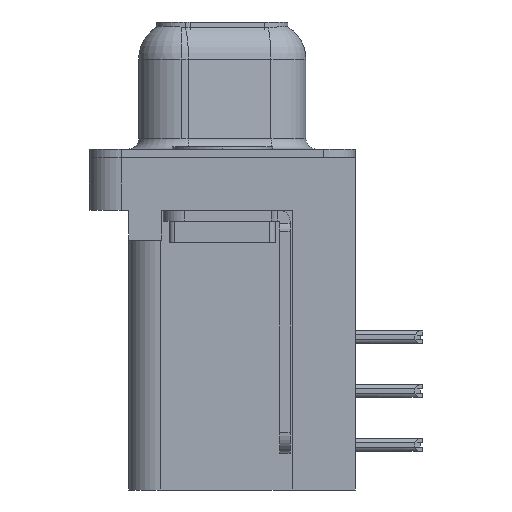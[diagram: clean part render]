
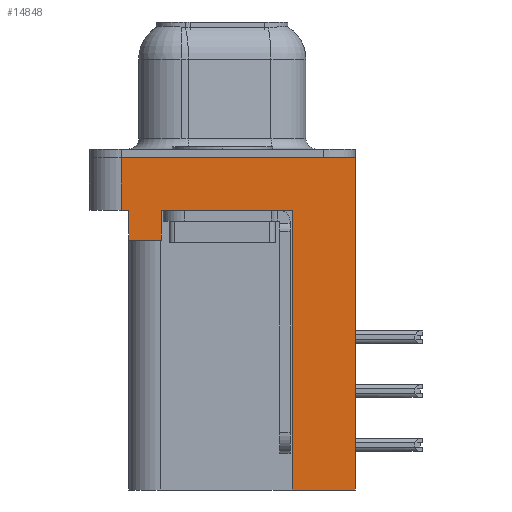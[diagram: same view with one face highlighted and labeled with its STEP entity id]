
A CAD part, left-side view. The second image highlights one B-rep face of the part: STEP entity #14848.
In plain terms, the highlighted planar face has unit normal (-1, 0, 0).
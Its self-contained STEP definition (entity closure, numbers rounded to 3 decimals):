
#446 = VECTOR ( 'NONE', #33375, 1000. ) ;
#2451 = DIRECTION ( 'NONE',  ( 0., 1., 0. ) ) ;
#3460 = ORIENTED_EDGE ( 'NONE', *, *, #33896, .F. ) ;
#3939 = DIRECTION ( 'NONE',  ( 0., 0., 1. ) ) ;
#4551 = CARTESIAN_POINT ( 'NONE',  ( -2.935, 4.425, -3.9 ) ) ;
#4789 = CARTESIAN_POINT ( 'NONE',  ( -2.935, -3.295, -15.7 ) ) ;
#4794 = EDGE_LOOP ( 'NONE', ( #4999, #20649, #5176, #29554, #32400, #23883, #32715, #3460, #33951, #23273 ) ) ;
#4872 = VECTOR ( 'NONE', #16156, 1000. ) ;
#4999 = ORIENTED_EDGE ( 'NONE', *, *, #17273, .F. ) ;
#5027 = AXIS2_PLACEMENT_3D ( 'NONE', #14839, #20171, #3939 ) ;
#5176 = ORIENTED_EDGE ( 'NONE', *, *, #31374, .T. ) ;
#6061 = VECTOR ( 'NONE', #17089, 1000. ) ;
#7099 = VECTOR ( 'NONE', #20869, 1000. ) ;
#8387 = CARTESIAN_POINT ( 'NONE',  ( -2.935, 2.895, -3.9 ) ) ;
#9916 = VECTOR ( 'NONE', #16179, 1000. ) ;
#9974 = DIRECTION ( 'NONE',  ( 0., 0., 1. ) ) ;
#12251 = VECTOR ( 'NONE', #33177, 1000. ) ;
#14275 = CARTESIAN_POINT ( 'NONE',  ( -2.935, 4.775, -2.5 ) ) ;
#14746 = LINE ( 'NONE', #4789, #27880 ) ;
#14839 = CARTESIAN_POINT ( 'NONE',  ( -2.935, -6.275, -2.5 ) ) ;
#14848 = ADVANCED_FACE ( 'NONE', ( #24553 ), #27920, .T. ) ;
#15179 = VERTEX_POINT ( 'NONE', #8387 ) ;
#15581 = VECTOR ( 'NONE', #9974, 1000. ) ;
#16058 = VERTEX_POINT ( 'NONE', #16353 ) ;
#16114 = VERTEX_POINT ( 'NONE', #30134 ) ;
#16156 = DIRECTION ( 'NONE',  ( 0., 0., 1. ) ) ;
#16179 = DIRECTION ( 'NONE',  ( 0., 0., 1. ) ) ;
#16353 = CARTESIAN_POINT ( 'NONE',  ( -2.935, 4.425, -2.5 ) ) ;
#16846 = CARTESIAN_POINT ( 'NONE',  ( -2.935, 4.775, 0. ) ) ;
#17089 = DIRECTION ( 'NONE',  ( 0., 0., 1. ) ) ;
#17180 = CARTESIAN_POINT ( 'NONE',  ( -2.935, -3.295, -15.7 ) ) ;
#17273 = EDGE_CURVE ( 'NONE', #19043, #19948, #26388, .T. ) ;
#18913 = CARTESIAN_POINT ( 'NONE',  ( -2.935, -3.295, -2.5 ) ) ;
#19043 = VERTEX_POINT ( 'NONE', #16846 ) ;
#19744 = LINE ( 'NONE', #31735, #25955 ) ;
#19948 = VERTEX_POINT ( 'NONE', #25061 ) ;
#20163 = LINE ( 'NONE', #29247, #4872 ) ;
#20171 = DIRECTION ( 'NONE',  ( -1., 0., 0. ) ) ;
#20406 = VERTEX_POINT ( 'NONE', #18913 ) ;
#20649 = ORIENTED_EDGE ( 'NONE', *, *, #33470, .F. ) ;
#20869 = DIRECTION ( 'NONE',  ( 0., -1., 0. ) ) ;
#21993 = LINE ( 'NONE', #30732, #446 ) ;
#22099 = CARTESIAN_POINT ( 'NONE',  ( -2.935, -6.275, -2.5 ) ) ;
#23273 = ORIENTED_EDGE ( 'NONE', *, *, #28441, .T. ) ;
#23883 = ORIENTED_EDGE ( 'NONE', *, *, #27947, .T. ) ;
#24311 = VECTOR ( 'NONE', #24794, 1000. ) ;
#24553 = FACE_OUTER_BOUND ( 'NONE', #4794, .T. ) ;
#24794 = DIRECTION ( 'NONE',  ( 0., -1., 0. ) ) ;
#24910 = CARTESIAN_POINT ( 'NONE',  ( -2.935, 4.425, -3.9 ) ) ;
#25061 = CARTESIAN_POINT ( 'NONE',  ( -2.935, -6.275, 0. ) ) ;
#25160 = LINE ( 'NONE', #31890, #9916 ) ;
#25955 = VECTOR ( 'NONE', #2451, 1000. ) ;
#26388 = LINE ( 'NONE', #30532, #12251 ) ;
#26442 = EDGE_CURVE ( 'NONE', #16114, #20406, #31959, .T. ) ;
#26483 = VERTEX_POINT ( 'NONE', #14275 ) ;
#26704 = VERTEX_POINT ( 'NONE', #17180 ) ;
#27106 = VERTEX_POINT ( 'NONE', #32365 ) ;
#27443 = LINE ( 'NONE', #27515, #6061 ) ;
#27515 = CARTESIAN_POINT ( 'NONE',  ( -2.935, 2.895, -3.9 ) ) ;
#27880 = VECTOR ( 'NONE', #34001, 1000. ) ;
#27920 = PLANE ( 'NONE',  #5027 ) ;
#27947 = EDGE_CURVE ( 'NONE', #15179, #16114, #27443, .T. ) ;
#28441 = EDGE_CURVE ( 'NONE', #27106, #19948, #25160, .T. ) ;
#29247 = CARTESIAN_POINT ( 'NONE',  ( -2.935, 4.775, -2.5 ) ) ;
#29529 = LINE ( 'NONE', #4551, #15581 ) ;
#29554 = ORIENTED_EDGE ( 'NONE', *, *, #33846, .F. ) ;
#30134 = CARTESIAN_POINT ( 'NONE',  ( -2.935, 2.895, -2.5 ) ) ;
#30304 = VERTEX_POINT ( 'NONE', #24910 ) ;
#30479 = EDGE_CURVE ( 'NONE', #15179, #30304, #21993, .T. ) ;
#30532 = CARTESIAN_POINT ( 'NONE',  ( -2.935, -6.275, 0. ) ) ;
#30732 = CARTESIAN_POINT ( 'NONE',  ( -2.935, 4.425, -3.9 ) ) ;
#30907 = LINE ( 'NONE', #31244, #7099 ) ;
#31244 = CARTESIAN_POINT ( 'NONE',  ( -2.935, -6.275, -2.5 ) ) ;
#31374 = EDGE_CURVE ( 'NONE', #26483, #16058, #30907, .T. ) ;
#31735 = CARTESIAN_POINT ( 'NONE',  ( -2.935, -3.295, -15.7 ) ) ;
#31890 = CARTESIAN_POINT ( 'NONE',  ( -2.935, -6.275, -2.5 ) ) ;
#31959 = LINE ( 'NONE', #22099, #24311 ) ;
#32365 = CARTESIAN_POINT ( 'NONE',  ( -2.935, -6.275, -15.7 ) ) ;
#32400 = ORIENTED_EDGE ( 'NONE', *, *, #30479, .F. ) ;
#32715 = ORIENTED_EDGE ( 'NONE', *, *, #26442, .T. ) ;
#33177 = DIRECTION ( 'NONE',  ( 0., -1., 0. ) ) ;
#33375 = DIRECTION ( 'NONE',  ( 0., 1., 0. ) ) ;
#33470 = EDGE_CURVE ( 'NONE', #26483, #19043, #20163, .T. ) ;
#33846 = EDGE_CURVE ( 'NONE', #30304, #16058, #29529, .T. ) ;
#33896 = EDGE_CURVE ( 'NONE', #26704, #20406, #14746, .T. ) ;
#33951 = ORIENTED_EDGE ( 'NONE', *, *, #33998, .F. ) ;
#33998 = EDGE_CURVE ( 'NONE', #27106, #26704, #19744, .T. ) ;
#34001 = DIRECTION ( 'NONE',  ( 0., 0., 1. ) ) ;
